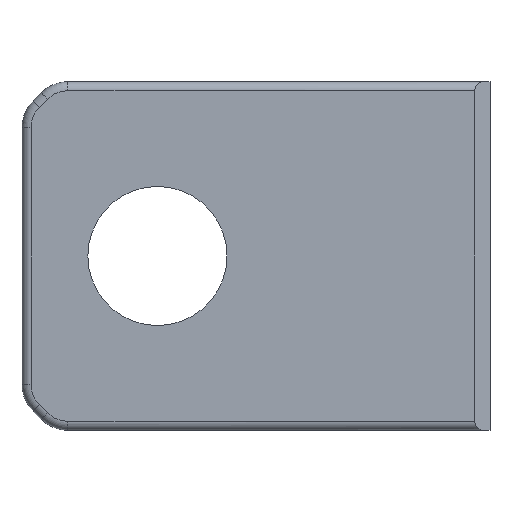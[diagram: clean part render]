
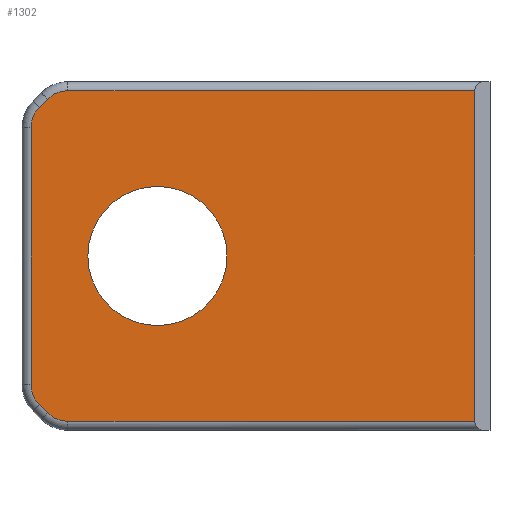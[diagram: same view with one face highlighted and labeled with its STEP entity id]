
A CAD part, front view. The second image highlights one B-rep face of the part: STEP entity #1302.
In plain terms, the highlighted planar face has unit normal (0, -1, 0).
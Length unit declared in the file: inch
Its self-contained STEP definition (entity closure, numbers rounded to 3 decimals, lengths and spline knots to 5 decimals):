
#31=FACE_BOUND('',#160,.T.);
#33=PLANE('',#1422);
#77=FACE_OUTER_BOUND('',#159,.T.);
#159=EDGE_LOOP('',(#882,#883,#884,#885,#886,#887,#888,#889,#890,#891));
#160=EDGE_LOOP('',(#892));
#237=CIRCLE('',#1401,0.095);
#241=CIRCLE('',#1407,0.095);
#245=CIRCLE('',#1413,0.095);
#249=CIRCLE('',#1419,0.095);
#250=CIRCLE('',#1423,0.23);
#312=LINE('',#2011,#410);
#315=LINE('',#2026,#413);
#317=LINE('',#2038,#415);
#319=LINE('',#2050,#417);
#321=LINE('',#2062,#419);
#322=LINE('',#2064,#420);
#410=VECTOR('',#1571,0.3937);
#413=VECTOR('',#1588,0.3937);
#415=VECTOR('',#1602,0.3937);
#417=VECTOR('',#1616,0.3937);
#419=VECTOR('',#1630,0.3937);
#420=VECTOR('',#1633,0.3937);
#523=VERTEX_POINT('',#2008);
#524=VERTEX_POINT('',#2010);
#526=VERTEX_POINT('',#2016);
#528=VERTEX_POINT('',#2022);
#530=VERTEX_POINT('',#2028);
#532=VERTEX_POINT('',#2034);
#534=VERTEX_POINT('',#2040);
#536=VERTEX_POINT('',#2046);
#538=VERTEX_POINT('',#2052);
#540=VERTEX_POINT('',#2058);
#542=VERTEX_POINT('',#2065);
#645=EDGE_CURVE('',#523,#524,#312,.T.);
#650=EDGE_CURVE('',#524,#526,#237,.T.);
#653=EDGE_CURVE('',#526,#528,#315,.T.);
#656=EDGE_CURVE('',#528,#530,#241,.T.);
#659=EDGE_CURVE('',#530,#532,#317,.T.);
#662=EDGE_CURVE('',#532,#534,#245,.T.);
#665=EDGE_CURVE('',#534,#536,#319,.T.);
#668=EDGE_CURVE('',#536,#538,#249,.T.);
#671=EDGE_CURVE('',#538,#540,#321,.T.);
#672=EDGE_CURVE('',#540,#523,#322,.T.);
#673=EDGE_CURVE('',#542,#542,#250,.F.);
#882=ORIENTED_EDGE('',*,*,#671,.F.);
#883=ORIENTED_EDGE('',*,*,#668,.F.);
#884=ORIENTED_EDGE('',*,*,#665,.F.);
#885=ORIENTED_EDGE('',*,*,#662,.F.);
#886=ORIENTED_EDGE('',*,*,#659,.F.);
#887=ORIENTED_EDGE('',*,*,#656,.F.);
#888=ORIENTED_EDGE('',*,*,#653,.F.);
#889=ORIENTED_EDGE('',*,*,#650,.F.);
#890=ORIENTED_EDGE('',*,*,#645,.F.);
#891=ORIENTED_EDGE('',*,*,#672,.F.);
#892=ORIENTED_EDGE('',*,*,#673,.T.);
#1302=ADVANCED_FACE('',(#77,#31),#33,.F.);
#1401=AXIS2_PLACEMENT_3D('',#2020,#1581,#1582);
#1407=AXIS2_PLACEMENT_3D('',#2032,#1595,#1596);
#1413=AXIS2_PLACEMENT_3D('',#2044,#1609,#1610);
#1419=AXIS2_PLACEMENT_3D('',#2056,#1623,#1624);
#1422=AXIS2_PLACEMENT_3D('',#2063,#1631,#1632);
#1423=AXIS2_PLACEMENT_3D('',#2066,#1634,#1635);
#1571=DIRECTION('',(-1.,0.,0.));
#1581=DIRECTION('center_axis',(0.,1.,0.));
#1582=DIRECTION('ref_axis',(-0.383,0.,-0.924));
#1588=DIRECTION('',(-0.707,0.,0.707));
#1595=DIRECTION('center_axis',(0.,1.,0.));
#1596=DIRECTION('ref_axis',(-0.924,0.,-0.383));
#1602=DIRECTION('',(0.,0.,1.));
#1609=DIRECTION('center_axis',(0.,1.,0.));
#1610=DIRECTION('ref_axis',(-0.924,0.,0.383));
#1616=DIRECTION('',(0.707,0.,0.707));
#1623=DIRECTION('center_axis',(0.,1.,0.));
#1624=DIRECTION('ref_axis',(-0.383,0.,0.924));
#1630=DIRECTION('',(1.,0.,0.));
#1631=DIRECTION('center_axis',(0.,1.,0.));
#1632=DIRECTION('ref_axis',(0.,0.,1.));
#1633=DIRECTION('',(0.,0.,-1.));
#1634=DIRECTION('center_axis',(0.,-1.,0.));
#1635=DIRECTION('ref_axis',(-1.,0.,0.));
#2008=CARTESIAN_POINT('',(1.498,-0.05,-1.113));
#2010=CARTESIAN_POINT('',(0.15178,-0.05,-1.113));
#2011=CARTESIAN_POINT('',(1.161,-0.05,-1.113));
#2016=CARTESIAN_POINT('',(0.0846,-0.05,-1.08518));
#2020=CARTESIAN_POINT('Origin',(0.15178,-0.05,-1.018));
#2022=CARTESIAN_POINT('',(0.05782,-0.05,-1.0584));
#2026=CARTESIAN_POINT('',(0.12059,-0.05,-1.12116));
#2028=CARTESIAN_POINT('',(0.03,-0.05,-0.99122));
#2032=CARTESIAN_POINT('Origin',(0.125,-0.05,-0.99122));
#2034=CARTESIAN_POINT('',(0.03,-0.05,-0.14178));
#2038=CARTESIAN_POINT('',(0.03,-0.05,-0.84975));
#2040=CARTESIAN_POINT('',(0.05782,-0.05,-0.0746));
#2044=CARTESIAN_POINT('Origin',(0.125,-0.05,-0.14178));
#2046=CARTESIAN_POINT('',(0.0846,-0.05,-0.04782));
#2050=CARTESIAN_POINT('',(0.12059,-0.05,-0.01184));
#2052=CARTESIAN_POINT('',(0.15178,-0.05,-0.02));
#2056=CARTESIAN_POINT('Origin',(0.15178,-0.05,-0.115));
#2058=CARTESIAN_POINT('',(1.498,-0.05,-0.02));
#2062=CARTESIAN_POINT('',(0.387,-0.05,-0.02));
#2063=CARTESIAN_POINT('Origin',(0.774,-0.05,-0.5665));
#2064=CARTESIAN_POINT('',(1.498,-0.05,-0.28325));
#2065=CARTESIAN_POINT('',(0.678,-0.05,-0.5665));
#2066=CARTESIAN_POINT('Origin',(0.448,-0.05,-0.5665));
